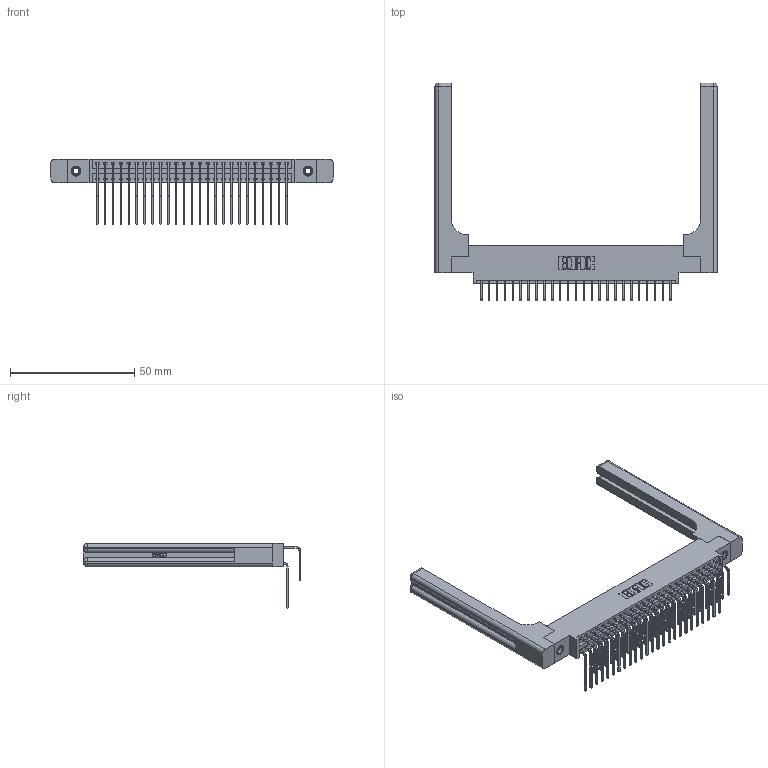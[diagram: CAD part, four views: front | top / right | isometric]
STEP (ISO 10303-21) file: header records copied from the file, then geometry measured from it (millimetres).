
FILE_DESCRIPTION (( 'STEP AP203' ), '1' );
FILE_NAME ('346-050-558-858.STEP', '2022-05-21T00:01:16', ( '' ), ( '' ), 'SwSTEP 2.0', 'SolidWorks 2020', '' );
FILE_SCHEMA (( 'CONFIG_CONTROL_DESIGN' ));
Length unit declared in the file: inch
Products named in the file (6): 346-220-058_345-220-058; 346-050-558-858; 345-292-001_558 559 Tail - 1; 345-292-001_558 Tail - 2; 346 Part_0.170 Offset - 0.156 Dia-TH; 345-250-001_345-250-001-102
Assembly tree (55 placements, depth 2):
  346-050-558-858
    346 Part_0.170 Offset - 0.156 Dia-TH
    345-292-001_558 559 Tail - 1  x25
    345-292-001_558 Tail - 2  x25
    345-250-001_345-250-001-102  x2
    346-220-058_345-220-058  x2
Bounding box: 113.44 x 87.44 x 26.16 mm (x, y, z)
Volume: 18539.4 mm3; surface area: 21485.8 mm2
Topology: 55 solids, 55 shells, 3096 faces, 9093 edges, 5974 vertices
Faces by surface type: plane 2092, cylinder 944, bspline 36, cone 12, sphere 8, torus 4
Entity records: 26118 total; most frequent: CARTESIAN_POINT 5394, ORIENTED_EDGE 4072, DIRECTION 3708, EDGE_CURVE 2036, LINE 1672, VECTOR 1672, VERTEX_POINT 1346, AXIS2_PLACEMENT_3D 1018
